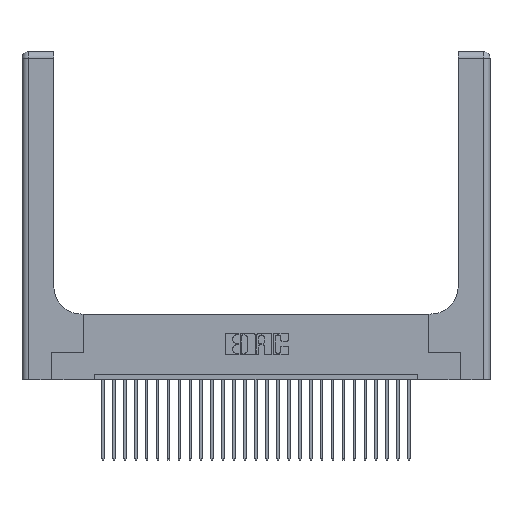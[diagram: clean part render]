
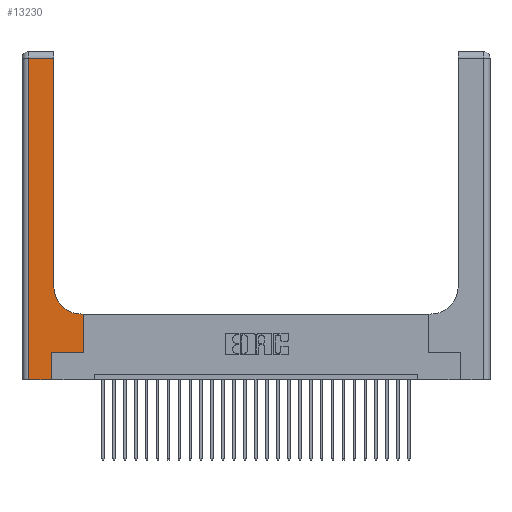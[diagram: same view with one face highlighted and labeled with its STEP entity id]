
A CAD part, top view. The second image highlights one B-rep face of the part: STEP entity #13230.
In plain terms, the highlighted planar face has unit normal (0, 0, 1).
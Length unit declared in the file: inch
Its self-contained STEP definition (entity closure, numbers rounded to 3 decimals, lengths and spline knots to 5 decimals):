
#10 = EDGE_CURVE ( 'NONE', #15617, #1956, #21575, .T. ) ;
#168 = CARTESIAN_POINT ( 'NONE',  ( 0.269, 0.25, 0.37 ) ) ;
#461 = DIRECTION ( 'NONE',  ( -1., 0., 0. ) ) ;
#586 = CARTESIAN_POINT ( 'NONE',  ( 0.2915, 0.85, 0.37 ) ) ;
#1605 = AXIS2_PLACEMENT_3D ( 'NONE', #15751, #6532, #8780 ) ;
#1850 = DIRECTION ( 'NONE',  ( 0., 1., 0. ) ) ;
#1956 = VERTEX_POINT ( 'NONE', #26063 ) ;
#2660 = DIRECTION ( 'NONE',  ( -1., 0., 0. ) ) ;
#2731 = ORIENTED_EDGE ( 'NONE', *, *, #25263, .T. ) ;
#2973 = DIRECTION ( 'NONE',  ( 0., 1., 0. ) ) ;
#3103 = VECTOR ( 'NONE', #5027, 39.37008 ) ;
#4403 = EDGE_CURVE ( 'NONE', #18809, #18333, #13241, .T. ) ;
#5027 = DIRECTION ( 'NONE',  ( 0., -1., 0. ) ) ;
#5443 = VERTEX_POINT ( 'NONE', #14673 ) ;
#5488 = ORIENTED_EDGE ( 'NONE', *, *, #14441, .T. ) ;
#6348 = FACE_OUTER_BOUND ( 'NONE', #27329, .T. ) ;
#6532 = DIRECTION ( 'NONE',  ( 0., 0., -1. ) ) ;
#6915 = VECTOR ( 'NONE', #16589, 39.37008 ) ;
#7070 = CARTESIAN_POINT ( 'NONE',  ( 0.06, 3., 0.37 ) ) ;
#7505 = VECTOR ( 'NONE', #1850, 39.37008 ) ;
#7866 = VERTEX_POINT ( 'NONE', #11926 ) ;
#8780 = DIRECTION ( 'NONE',  ( 1., 0., 0. ) ) ;
#9605 = LINE ( 'NONE', #11798, #27651 ) ;
#9714 = ORIENTED_EDGE ( 'NONE', *, *, #10149, .T. ) ;
#10149 = EDGE_CURVE ( 'NONE', #19095, #15617, #25384, .T. ) ;
#10793 = ORIENTED_EDGE ( 'NONE', *, *, #4403, .T. ) ;
#11237 = VECTOR ( 'NONE', #28726, 39.37008 ) ;
#11798 = CARTESIAN_POINT ( 'NONE',  ( 0.269, 0., 0.37 ) ) ;
#11922 = PLANE ( 'NONE',  #16286 ) ;
#11926 = CARTESIAN_POINT ( 'NONE',  ( 0.5585, 0.6, 0.37 ) ) ;
#12185 = DIRECTION ( 'NONE',  ( 0., 1., 0. ) ) ;
#12310 = CARTESIAN_POINT ( 'NONE',  ( 0.2915, 2.94, 0.37 ) ) ;
#12691 = LINE ( 'NONE', #22060, #7505 ) ;
#12867 = EDGE_CURVE ( 'NONE', #16626, #16231, #16114, .T. ) ;
#13230 = ADVANCED_FACE ( 'NONE', ( #6348 ), #11922, .F. ) ;
#13241 = LINE ( 'NONE', #20690, #16731 ) ;
#13283 = CARTESIAN_POINT ( 'NONE',  ( 0., 2.94, 0.37 ) ) ;
#13721 = CARTESIAN_POINT ( 'NONE',  ( 0.2915, 0.6, 0.37 ) ) ;
#13764 = DIRECTION ( 'NONE',  ( 0., 0., -1. ) ) ;
#13781 = LINE ( 'NONE', #13721, #23936 ) ;
#14441 = EDGE_CURVE ( 'NONE', #1956, #16626, #9605, .T. ) ;
#14673 = CARTESIAN_POINT ( 'NONE',  ( 0.5415, 0.6, 0.37 ) ) ;
#15158 = ORIENTED_EDGE ( 'NONE', *, *, #10, .T. ) ;
#15617 = VERTEX_POINT ( 'NONE', #22959 ) ;
#15751 = CARTESIAN_POINT ( 'NONE',  ( 0.5415, 0.85, 0.37 ) ) ;
#15902 = CARTESIAN_POINT ( 'NONE',  ( 0., 3., 0.37 ) ) ;
#15979 = CARTESIAN_POINT ( 'NONE',  ( 0., 0., 0.37 ) ) ;
#16114 = LINE ( 'NONE', #168, #11237 ) ;
#16231 = VERTEX_POINT ( 'NONE', #28545 ) ;
#16286 = AXIS2_PLACEMENT_3D ( 'NONE', #15902, #13764, #18163 ) ;
#16589 = DIRECTION ( 'NONE',  ( 1., 0., 0. ) ) ;
#16626 = VERTEX_POINT ( 'NONE', #28233 ) ;
#16731 = VECTOR ( 'NONE', #2973, 39.37008 ) ;
#16759 = ORIENTED_EDGE ( 'NONE', *, *, #20522, .T. ) ;
#17455 = ORIENTED_EDGE ( 'NONE', *, *, #12867, .T. ) ;
#17952 = CIRCLE ( 'NONE', #1605, 0.25 ) ;
#18163 = DIRECTION ( 'NONE',  ( -1., 0., 0. ) ) ;
#18333 = VERTEX_POINT ( 'NONE', #12310 ) ;
#18809 = VERTEX_POINT ( 'NONE', #586 ) ;
#19083 = VECTOR ( 'NONE', #461, 39.37008 ) ;
#19095 = VERTEX_POINT ( 'NONE', #20248 ) ;
#20248 = CARTESIAN_POINT ( 'NONE',  ( 0.06, 2.94, 0.37 ) ) ;
#20522 = EDGE_CURVE ( 'NONE', #7866, #5443, #13781, .T. ) ;
#20690 = CARTESIAN_POINT ( 'NONE',  ( 0.2915, 3., 0.37 ) ) ;
#21575 = LINE ( 'NONE', #15979, #6915 ) ;
#22060 = CARTESIAN_POINT ( 'NONE',  ( 0.5585, 0.25, 0.37 ) ) ;
#22959 = CARTESIAN_POINT ( 'NONE',  ( 0.06, 0., 0.37 ) ) ;
#23712 = EDGE_CURVE ( 'NONE', #18333, #19095, #28094, .T. ) ;
#23936 = VECTOR ( 'NONE', #2660, 39.37008 ) ;
#24810 = ORIENTED_EDGE ( 'NONE', *, *, #23712, .T. ) ;
#25263 = EDGE_CURVE ( 'NONE', #5443, #18809, #17952, .T. ) ;
#25309 = ORIENTED_EDGE ( 'NONE', *, *, #25667, .T. ) ;
#25384 = LINE ( 'NONE', #7070, #3103 ) ;
#25667 = EDGE_CURVE ( 'NONE', #16231, #7866, #12691, .T. ) ;
#26063 = CARTESIAN_POINT ( 'NONE',  ( 0.269, 0., 0.37 ) ) ;
#27329 = EDGE_LOOP ( 'NONE', ( #10793, #24810, #9714, #15158, #5488, #17455, #25309, #16759, #2731 ) ) ;
#27651 = VECTOR ( 'NONE', #12185, 39.37008 ) ;
#28094 = LINE ( 'NONE', #13283, #19083 ) ;
#28233 = CARTESIAN_POINT ( 'NONE',  ( 0.269, 0.25, 0.37 ) ) ;
#28545 = CARTESIAN_POINT ( 'NONE',  ( 0.5585, 0.25, 0.37 ) ) ;
#28726 = DIRECTION ( 'NONE',  ( 1., 0., 0. ) ) ;
